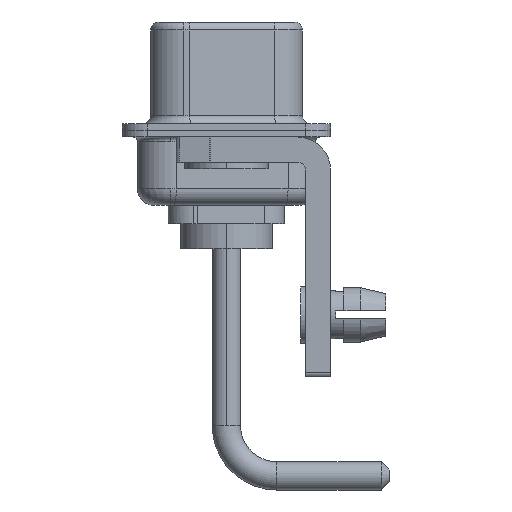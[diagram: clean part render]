
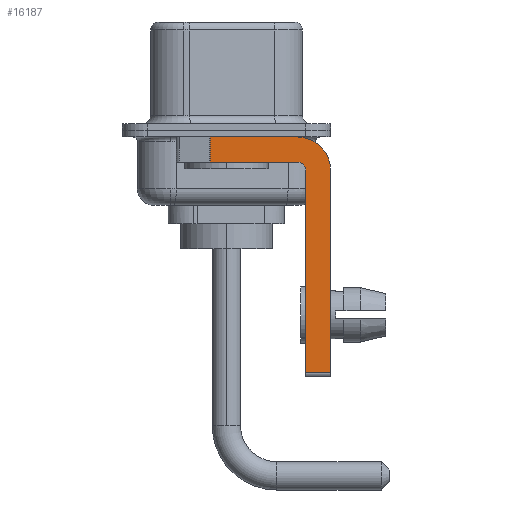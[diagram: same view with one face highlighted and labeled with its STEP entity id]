
A CAD part, left-side view. The second image highlights one B-rep face of the part: STEP entity #16187.
In plain terms, the highlighted planar face has unit normal (-1, 0, 0).
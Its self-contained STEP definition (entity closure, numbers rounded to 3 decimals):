
#458 = CARTESIAN_POINT ( 'NONE',  ( -2.9, -4.75, -2.4 ) ) ;
#514 = CARTESIAN_POINT ( 'NONE',  ( -2.9, -4.25, -2.4 ) ) ;
#951 = CARTESIAN_POINT ( 'NONE',  ( -2.9, 3., -0.4 ) ) ;
#1303 = CARTESIAN_POINT ( 'NONE',  ( -2.9, 0.978, -1.9 ) ) ;
#1866 = DIRECTION ( 'NONE',  ( 0., 0., -1. ) ) ;
#1874 = FACE_OUTER_BOUND ( 'NONE', #9206, .T. ) ;
#1876 = EDGE_CURVE ( 'NONE', #8047, #11551, #12026, .T. ) ;
#1888 = ORIENTED_EDGE ( 'NONE', *, *, #3712, .F. ) ;
#1984 = EDGE_CURVE ( 'NONE', #14192, #5805, #6943, .T. ) ;
#2053 = CARTESIAN_POINT ( 'NONE',  ( -2.9, 0.978, -1.9 ) ) ;
#2609 = ORIENTED_EDGE ( 'NONE', *, *, #4521, .T. ) ;
#2640 = ORIENTED_EDGE ( 'NONE', *, *, #14910, .F. ) ;
#3079 = CARTESIAN_POINT ( 'NONE',  ( -2.9, -4.25, -2.4 ) ) ;
#3507 = CARTESIAN_POINT ( 'NONE',  ( -2.9, -6.25, -14.55 ) ) ;
#3567 = VERTEX_POINT ( 'NONE', #458 ) ;
#3684 = DIRECTION ( 'NONE',  ( 0., -1., 0. ) ) ;
#3712 = EDGE_CURVE ( 'NONE', #12370, #10784, #10298, .T. ) ;
#3912 = ORIENTED_EDGE ( 'NONE', *, *, #1984, .F. ) ;
#4110 = CARTESIAN_POINT ( 'NONE',  ( -2.9, -4.75, -14.55 ) ) ;
#4359 = CARTESIAN_POINT ( 'NONE',  ( -2.9, -4.25, -2.4 ) ) ;
#4513 = CARTESIAN_POINT ( 'NONE',  ( -2.9, -6.25, -2.4 ) ) ;
#4521 = EDGE_CURVE ( 'NONE', #12370, #5805, #4600, .T. ) ;
#4539 = ORIENTED_EDGE ( 'NONE', *, *, #8696, .F. ) ;
#4598 = DIRECTION ( 'NONE',  ( 0., 0., -1. ) ) ;
#4600 = LINE ( 'NONE', #2053, #15981 ) ;
#4689 = DIRECTION ( 'NONE',  ( 0., 0., -1. ) ) ;
#4715 = LINE ( 'NONE', #12353, #14912 ) ;
#5482 = DIRECTION ( 'NONE',  ( 0., -1., 0. ) ) ;
#5805 = VERTEX_POINT ( 'NONE', #1303 ) ;
#5871 = PLANE ( 'NONE',  #8713 ) ;
#5879 = DIRECTION ( 'NONE',  ( 0., 0., -1. ) ) ;
#5897 = DIRECTION ( 'NONE',  ( 0., 0., 1. ) ) ;
#6655 = EDGE_CURVE ( 'NONE', #10784, #8770, #9779, .T. ) ;
#6943 = LINE ( 'NONE', #12350, #14833 ) ;
#6984 = CARTESIAN_POINT ( 'NONE',  ( -2.9, -6.25, -2.4 ) ) ;
#7081 = DIRECTION ( 'NONE',  ( 1., 0., 0. ) ) ;
#7332 = ORIENTED_EDGE ( 'NONE', *, *, #1876, .T. ) ;
#7484 = ORIENTED_EDGE ( 'NONE', *, *, #7750, .F. ) ;
#7600 = AXIS2_PLACEMENT_3D ( 'NONE', #514, #8253, #12392 ) ;
#7750 = EDGE_CURVE ( 'NONE', #8047, #3567, #4715, .T. ) ;
#8047 = VERTEX_POINT ( 'NONE', #4110 ) ;
#8253 = DIRECTION ( 'NONE',  ( -1., 0., 0. ) ) ;
#8296 = ORIENTED_EDGE ( 'NONE', *, *, #6655, .F. ) ;
#8438 = DIRECTION ( 'NONE',  ( 0., 1., 0. ) ) ;
#8696 = EDGE_CURVE ( 'NONE', #8770, #11551, #16141, .T. ) ;
#8713 = AXIS2_PLACEMENT_3D ( 'NONE', #3079, #13667, #4598 ) ;
#8770 = VERTEX_POINT ( 'NONE', #6984 ) ;
#9206 = EDGE_LOOP ( 'NONE', ( #1888, #2609, #3912, #2640, #7484, #7332, #4539, #8296 ) ) ;
#9239 = AXIS2_PLACEMENT_3D ( 'NONE', #4359, #7081, #5879 ) ;
#9393 = CARTESIAN_POINT ( 'NONE',  ( -2.9, -4.25, -14.55 ) ) ;
#9779 = CIRCLE ( 'NONE', #9239, 2. ) ;
#10298 = LINE ( 'NONE', #951, #16482 ) ;
#10784 = VERTEX_POINT ( 'NONE', #13990 ) ;
#11182 = CARTESIAN_POINT ( 'NONE',  ( -2.9, 0.978, -0.4 ) ) ;
#11551 = VERTEX_POINT ( 'NONE', #3507 ) ;
#12026 = LINE ( 'NONE', #9393, #13312 ) ;
#12350 = CARTESIAN_POINT ( 'NONE',  ( -2.9, -4.25, -1.9 ) ) ;
#12353 = CARTESIAN_POINT ( 'NONE',  ( -2.9, -4.75, -14.8 ) ) ;
#12370 = VERTEX_POINT ( 'NONE', #11182 ) ;
#12392 = DIRECTION ( 'NONE',  ( 0., 0., 1. ) ) ;
#13312 = VECTOR ( 'NONE', #5482, 1000. ) ;
#13626 = CARTESIAN_POINT ( 'NONE',  ( -2.9, -4.25, -1.9 ) ) ;
#13667 = DIRECTION ( 'NONE',  ( 1., 0., 0. ) ) ;
#13842 = VECTOR ( 'NONE', #1866, 1000. ) ;
#13990 = CARTESIAN_POINT ( 'NONE',  ( -2.9, -4.25, -0.4 ) ) ;
#14192 = VERTEX_POINT ( 'NONE', #13626 ) ;
#14833 = VECTOR ( 'NONE', #8438, 1000. ) ;
#14903 = CIRCLE ( 'NONE', #7600, 0.5 ) ;
#14910 = EDGE_CURVE ( 'NONE', #3567, #14192, #14903, .T. ) ;
#14912 = VECTOR ( 'NONE', #5897, 1000. ) ;
#15981 = VECTOR ( 'NONE', #4689, 1000. ) ;
#16141 = LINE ( 'NONE', #4513, #13842 ) ;
#16187 = ADVANCED_FACE ( 'NONE', ( #1874 ), #5871, .F. ) ;
#16482 = VECTOR ( 'NONE', #3684, 1000. ) ;
